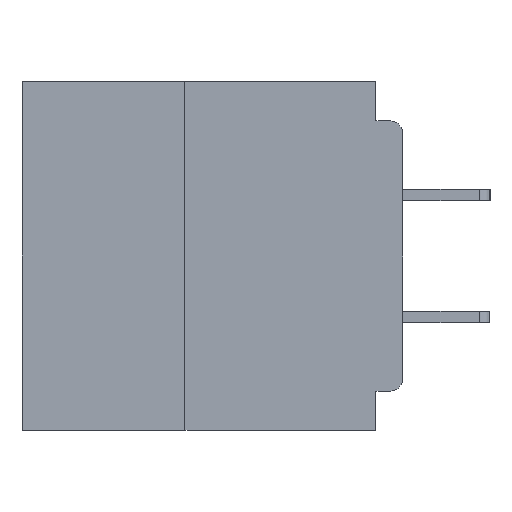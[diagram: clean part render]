
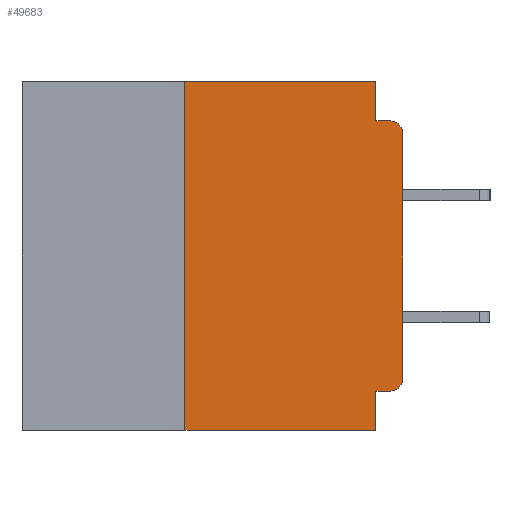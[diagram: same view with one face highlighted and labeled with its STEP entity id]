
A CAD part, left-side view. The second image highlights one B-rep face of the part: STEP entity #49683.
In plain terms, the highlighted planar face has unit normal (-1, 0, 0).
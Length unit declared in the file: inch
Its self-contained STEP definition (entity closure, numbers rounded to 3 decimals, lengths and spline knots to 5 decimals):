
#292 = CARTESIAN_POINT ( 'NONE',  ( 0., 0.437, 0. ) ) ;
#895 = ORIENTED_EDGE ( 'NONE', *, *, #59750, .T. ) ;
#991 = CARTESIAN_POINT ( 'NONE',  ( 0., 0.031, 0. ) ) ;
#2956 = DIRECTION ( 'NONE',  ( -1., 0., 0. ) ) ;
#3023 = CARTESIAN_POINT ( 'NONE',  ( 0., 0., -0.355 ) ) ;
#3979 = VECTOR ( 'NONE', #34915, 39.37008 ) ;
#4034 = CARTESIAN_POINT ( 'NONE',  ( 0., 0.25, -0.4 ) ) ;
#4816 = AXIS2_PLACEMENT_3D ( 'NONE', #35183, #2956, #40563 ) ;
#6128 = VECTOR ( 'NONE', #47060, 39.37008 ) ;
#6172 = CARTESIAN_POINT ( 'NONE',  ( 0., 0., 0. ) ) ;
#6767 = ORIENTED_EDGE ( 'NONE', *, *, #54801, .F. ) ;
#7839 = ORIENTED_EDGE ( 'NONE', *, *, #49776, .T. ) ;
#11557 = DIRECTION ( 'NONE',  ( 0., 0., 1. ) ) ;
#12330 = AXIS2_PLACEMENT_3D ( 'NONE', #27152, #64387, #32536 ) ;
#13643 = ORIENTED_EDGE ( 'NONE', *, *, #61285, .F. ) ;
#14609 = VERTEX_POINT ( 'NONE', #46143 ) ;
#14868 = VECTOR ( 'NONE', #28910, 39.37008 ) ;
#18248 = ORIENTED_EDGE ( 'NONE', *, *, #44307, .F. ) ;
#18464 = FACE_OUTER_BOUND ( 'NONE', #46734, .T. ) ;
#21312 = VERTEX_POINT ( 'NONE', #64829 ) ;
#21509 = PLANE ( 'NONE',  #46241 ) ;
#23299 = ORIENTED_EDGE ( 'NONE', *, *, #43803, .F. ) ;
#23668 = VECTOR ( 'NONE', #26124, 39.37008 ) ;
#24445 = DIRECTION ( 'NONE',  ( 0., 1., 0. ) ) ;
#24459 = EDGE_CURVE ( 'NONE', #59149, #21312, #28018, .T. ) ;
#24869 = ORIENTED_EDGE ( 'NONE', *, *, #24459, .T. ) ;
#24924 = CARTESIAN_POINT ( 'NONE',  ( 0., 0., -0.06 ) ) ;
#25806 = LINE ( 'NONE', #60814, #14868 ) ;
#26124 = DIRECTION ( 'NONE',  ( 0., 0., -1. ) ) ;
#26821 = VERTEX_POINT ( 'NONE', #47197 ) ;
#27152 = CARTESIAN_POINT ( 'NONE',  ( 0., 0.015, -0.34 ) ) ;
#27204 = DIRECTION ( 'NONE',  ( 0., -1., 0. ) ) ;
#27950 = VECTOR ( 'NONE', #24445, 39.37008 ) ;
#28018 = CIRCLE ( 'NONE', #4816, 0.015 ) ;
#28910 = DIRECTION ( 'NONE',  ( 0., -1., 0. ) ) ;
#29538 = CARTESIAN_POINT ( 'NONE',  ( 0., 0.031, 0. ) ) ;
#30257 = LINE ( 'NONE', #292, #67600 ) ;
#30504 = VECTOR ( 'NONE', #66661, 39.37008 ) ;
#32292 = DIRECTION ( 'NONE',  ( 0., 0., -1. ) ) ;
#32536 = DIRECTION ( 'NONE',  ( 0., 0., -1. ) ) ;
#34890 = CARTESIAN_POINT ( 'NONE',  ( 0., 0., -0.045 ) ) ;
#34915 = DIRECTION ( 'NONE',  ( 0., 0., -1. ) ) ;
#34931 = CIRCLE ( 'NONE', #12330, 0.015 ) ;
#35183 = CARTESIAN_POINT ( 'NONE',  ( 0., 0.015, -0.06 ) ) ;
#36172 = VERTEX_POINT ( 'NONE', #66925 ) ;
#36301 = CARTESIAN_POINT ( 'NONE',  ( 0., 0.25, -0.4 ) ) ;
#38884 = VERTEX_POINT ( 'NONE', #56524 ) ;
#39106 = EDGE_CURVE ( 'NONE', #38884, #58655, #66138, .T. ) ;
#40275 = LINE ( 'NONE', #6172, #66788 ) ;
#40563 = DIRECTION ( 'NONE',  ( 0., 0., -1. ) ) ;
#40932 = CARTESIAN_POINT ( 'NONE',  ( 0., 0.031, -0.4 ) ) ;
#41041 = ORIENTED_EDGE ( 'NONE', *, *, #66143, .F. ) ;
#42194 = LINE ( 'NONE', #3023, #27950 ) ;
#42291 = CARTESIAN_POINT ( 'NONE',  ( 0., 0.031, -0.4 ) ) ;
#43803 = EDGE_CURVE ( 'NONE', #52869, #14609, #61352, .T. ) ;
#44307 = EDGE_CURVE ( 'NONE', #26821, #38884, #42194, .T. ) ;
#45839 = VERTEX_POINT ( 'NONE', #991 ) ;
#46143 = CARTESIAN_POINT ( 'NONE',  ( 0., 0.25, 0. ) ) ;
#46241 = AXIS2_PLACEMENT_3D ( 'NONE', #58872, #64153, #32292 ) ;
#46479 = LINE ( 'NONE', #34890, #30504 ) ;
#46734 = EDGE_LOOP ( 'NONE', ( #7839, #24869, #13643, #41041, #6767, #23299, #52124, #64833, #18248, #895 ) ) ;
#47060 = DIRECTION ( 'NONE',  ( 0., 0., 1. ) ) ;
#47197 = CARTESIAN_POINT ( 'NONE',  ( 0., 0.015, -0.355 ) ) ;
#49683 = ADVANCED_FACE ( 'NONE', ( #18464 ), #21509, .F. ) ;
#49776 = EDGE_CURVE ( 'NONE', #68770, #59149, #40275, .T. ) ;
#52124 = ORIENTED_EDGE ( 'NONE', *, *, #67315, .T. ) ;
#52869 = VERTEX_POINT ( 'NONE', #36301 ) ;
#54801 = EDGE_CURVE ( 'NONE', #14609, #45839, #30257, .T. ) ;
#56524 = CARTESIAN_POINT ( 'NONE',  ( 0., 0.031, -0.355 ) ) ;
#56576 = CARTESIAN_POINT ( 'NONE',  ( 0., 0., -0.34 ) ) ;
#58655 = VERTEX_POINT ( 'NONE', #40932 ) ;
#58872 = CARTESIAN_POINT ( 'NONE',  ( 0., 0.437, 0. ) ) ;
#59149 = VERTEX_POINT ( 'NONE', #24924 ) ;
#59750 = EDGE_CURVE ( 'NONE', #26821, #68770, #34931, .T. ) ;
#60814 = CARTESIAN_POINT ( 'NONE',  ( 0., 0.437, -0.4 ) ) ;
#60928 = LINE ( 'NONE', #29538, #3979 ) ;
#61285 = EDGE_CURVE ( 'NONE', #36172, #21312, #46479, .T. ) ;
#61352 = LINE ( 'NONE', #4034, #6128 ) ;
#64153 = DIRECTION ( 'NONE',  ( 1., 0., 0. ) ) ;
#64387 = DIRECTION ( 'NONE',  ( -1., 0., 0. ) ) ;
#64829 = CARTESIAN_POINT ( 'NONE',  ( 0., 0.015, -0.045 ) ) ;
#64833 = ORIENTED_EDGE ( 'NONE', *, *, #39106, .F. ) ;
#66138 = LINE ( 'NONE', #42291, #23668 ) ;
#66143 = EDGE_CURVE ( 'NONE', #45839, #36172, #60928, .T. ) ;
#66661 = DIRECTION ( 'NONE',  ( 0., -1., 0. ) ) ;
#66788 = VECTOR ( 'NONE', #11557, 39.37008 ) ;
#66925 = CARTESIAN_POINT ( 'NONE',  ( 0., 0.031, -0.045 ) ) ;
#67315 = EDGE_CURVE ( 'NONE', #52869, #58655, #25806, .T. ) ;
#67600 = VECTOR ( 'NONE', #27204, 39.37008 ) ;
#68770 = VERTEX_POINT ( 'NONE', #56576 ) ;
